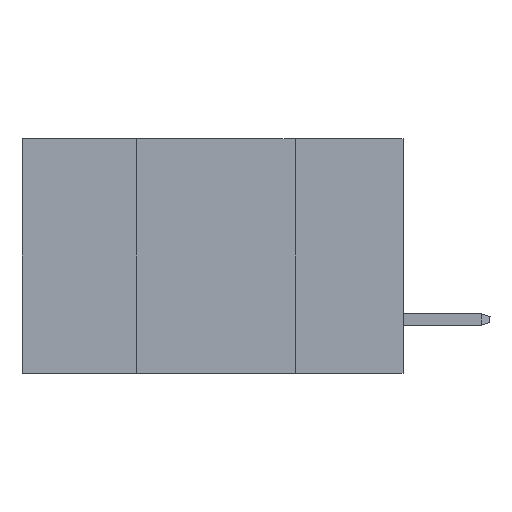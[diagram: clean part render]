
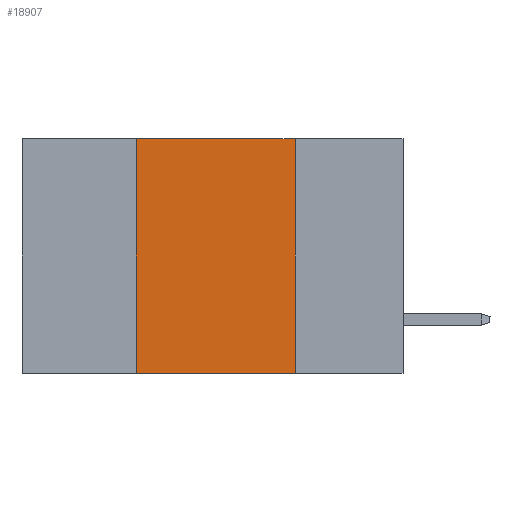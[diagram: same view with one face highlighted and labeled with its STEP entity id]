
A CAD part, left-side view. The second image highlights one B-rep face of the part: STEP entity #18907.
In plain terms, the highlighted planar face has unit normal (-1, 0, 0).
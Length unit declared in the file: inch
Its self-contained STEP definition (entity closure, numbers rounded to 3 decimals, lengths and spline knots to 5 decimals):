
#4 = VERTEX_POINT ( 'NONE', #23320 ) ;
#2094 = EDGE_CURVE ( 'NONE', #20901, #6405, #9575, .T. ) ;
#2514 = VERTEX_POINT ( 'NONE', #3630 ) ;
#3630 = CARTESIAN_POINT ( 'NONE',  ( 0., 0.17, -0.37 ) ) ;
#4056 = VECTOR ( 'NONE', #22383, 39.37008 ) ;
#4598 = EDGE_CURVE ( 'NONE', #6405, #4, #5307, .T. ) ;
#4686 = EDGE_CURVE ( 'NONE', #4, #2514, #13357, .T. ) ;
#4825 = CARTESIAN_POINT ( 'NONE',  ( 0., 0.42, -0.37 ) ) ;
#5307 = LINE ( 'NONE', #19978, #14046 ) ;
#5479 = ORIENTED_EDGE ( 'NONE', *, *, #2094, .F. ) ;
#5627 = DIRECTION ( 'NONE',  ( 0., -1., 0. ) ) ;
#6405 = VERTEX_POINT ( 'NONE', #19720 ) ;
#6688 = DIRECTION ( 'NONE',  ( 0., 0., 1. ) ) ;
#6980 = ORIENTED_EDGE ( 'NONE', *, *, #4686, .F. ) ;
#7716 = ORIENTED_EDGE ( 'NONE', *, *, #22740, .T. ) ;
#8087 = EDGE_LOOP ( 'NONE', ( #6980, #9467, #5479, #7716 ) ) ;
#8273 = CARTESIAN_POINT ( 'NONE',  ( 0., 0.42, 0. ) ) ;
#8409 = VECTOR ( 'NONE', #6688, 39.37008 ) ;
#9467 = ORIENTED_EDGE ( 'NONE', *, *, #4598, .F. ) ;
#9575 = LINE ( 'NONE', #8273, #8409 ) ;
#11063 = DIRECTION ( 'NONE',  ( 0., -1., 0. ) ) ;
#13301 = PLANE ( 'NONE',  #14521 ) ;
#13357 = LINE ( 'NONE', #20689, #4056 ) ;
#14046 = VECTOR ( 'NONE', #11063, 39.37008 ) ;
#14521 = AXIS2_PLACEMENT_3D ( 'NONE', #22934, #21003, #22575 ) ;
#14882 = CARTESIAN_POINT ( 'NONE',  ( 0., 0.6, -0.37 ) ) ;
#17506 = FACE_OUTER_BOUND ( 'NONE', #8087, .T. ) ;
#18375 = LINE ( 'NONE', #14882, #21972 ) ;
#18907 = ADVANCED_FACE ( 'NONE', ( #17506 ), #13301, .F. ) ;
#19720 = CARTESIAN_POINT ( 'NONE',  ( 0., 0.42, 0. ) ) ;
#19978 = CARTESIAN_POINT ( 'NONE',  ( 0., 0.6, 0. ) ) ;
#20689 = CARTESIAN_POINT ( 'NONE',  ( 0., 0.17, 0. ) ) ;
#20901 = VERTEX_POINT ( 'NONE', #4825 ) ;
#21003 = DIRECTION ( 'NONE',  ( 1., 0., 0. ) ) ;
#21972 = VECTOR ( 'NONE', #5627, 39.37008 ) ;
#22383 = DIRECTION ( 'NONE',  ( 0., 0., -1. ) ) ;
#22575 = DIRECTION ( 'NONE',  ( 0., 0., -1. ) ) ;
#22740 = EDGE_CURVE ( 'NONE', #20901, #2514, #18375, .T. ) ;
#22934 = CARTESIAN_POINT ( 'NONE',  ( 0., 0.6, 0. ) ) ;
#23320 = CARTESIAN_POINT ( 'NONE',  ( 0., 0.17, 0. ) ) ;
